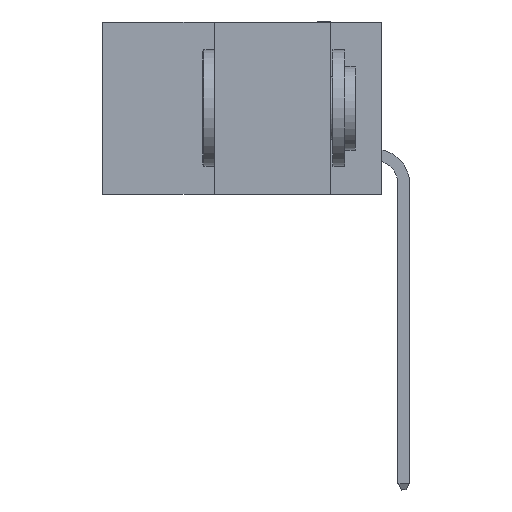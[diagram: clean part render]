
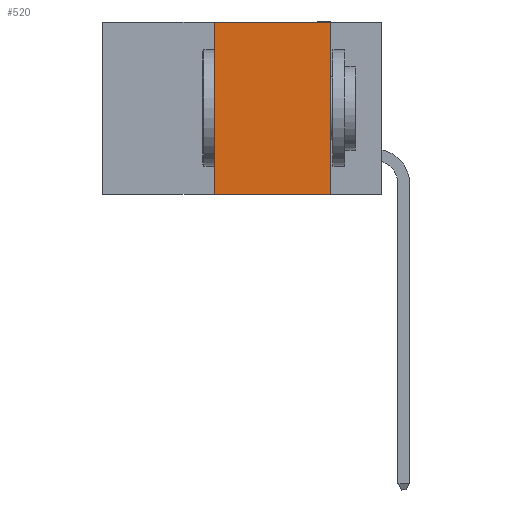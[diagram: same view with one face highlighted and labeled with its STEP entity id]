
A CAD part, left-side view. The second image highlights one B-rep face of the part: STEP entity #520.
In plain terms, the highlighted planar face has unit normal (-1, 0, 0).
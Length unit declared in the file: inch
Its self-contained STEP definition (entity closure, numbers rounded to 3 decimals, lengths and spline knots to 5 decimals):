
#33 = VECTOR ( 'NONE', #3476, 39.37008 ) ;
#520 = ADVANCED_FACE ( 'NONE', ( #874 ), #20718, .F. ) ;
#874 = FACE_OUTER_BOUND ( 'NONE', #17582, .T. ) ;
#1831 = EDGE_CURVE ( 'NONE', #6758, #14218, #6035, .T. ) ;
#2792 = CARTESIAN_POINT ( 'NONE',  ( 0., 0.6, 0. ) ) ;
#3294 = DIRECTION ( 'NONE',  ( 0., 0., -1. ) ) ;
#3476 = DIRECTION ( 'NONE',  ( 0., 0., 1. ) ) ;
#3549 = CARTESIAN_POINT ( 'NONE',  ( 0., 0.36, 0. ) ) ;
#5168 = VECTOR ( 'NONE', #14401, 39.37008 ) ;
#5450 = CARTESIAN_POINT ( 'NONE',  ( 0., 0.6, -0.37 ) ) ;
#6035 = LINE ( 'NONE', #3549, #33 ) ;
#6758 = VERTEX_POINT ( 'NONE', #16211 ) ;
#6889 = DIRECTION ( 'NONE',  ( 0., -1., 0. ) ) ;
#7067 = LINE ( 'NONE', #20879, #9161 ) ;
#7199 = ORIENTED_EDGE ( 'NONE', *, *, #16584, .F. ) ;
#7770 = CARTESIAN_POINT ( 'NONE',  ( 0., 0.6, 0. ) ) ;
#8630 = CARTESIAN_POINT ( 'NONE',  ( 0., 0.11, 0. ) ) ;
#9161 = VECTOR ( 'NONE', #3294, 39.37008 ) ;
#9444 = CARTESIAN_POINT ( 'NONE',  ( 0., 0.36, 0. ) ) ;
#10994 = DIRECTION ( 'NONE',  ( 0., 0., -1. ) ) ;
#13153 = EDGE_CURVE ( 'NONE', #16116, #20457, #7067, .T. ) ;
#13421 = LINE ( 'NONE', #5450, #20558 ) ;
#14218 = VERTEX_POINT ( 'NONE', #9444 ) ;
#14401 = DIRECTION ( 'NONE',  ( 0., -1., 0. ) ) ;
#14456 = AXIS2_PLACEMENT_3D ( 'NONE', #7770, #15873, #10994 ) ;
#15873 = DIRECTION ( 'NONE',  ( 1., 0., 0. ) ) ;
#16116 = VERTEX_POINT ( 'NONE', #8630 ) ;
#16211 = CARTESIAN_POINT ( 'NONE',  ( 0., 0.36, -0.37 ) ) ;
#16520 = ORIENTED_EDGE ( 'NONE', *, *, #1831, .F. ) ;
#16584 = EDGE_CURVE ( 'NONE', #14218, #16116, #19816, .T. ) ;
#16678 = EDGE_CURVE ( 'NONE', #6758, #20457, #13421, .T. ) ;
#17582 = EDGE_LOOP ( 'NONE', ( #18427, #7199, #16520, #18396 ) ) ;
#17916 = CARTESIAN_POINT ( 'NONE',  ( 0., 0.11, -0.37 ) ) ;
#18396 = ORIENTED_EDGE ( 'NONE', *, *, #16678, .T. ) ;
#18427 = ORIENTED_EDGE ( 'NONE', *, *, #13153, .F. ) ;
#19816 = LINE ( 'NONE', #2792, #5168 ) ;
#20457 = VERTEX_POINT ( 'NONE', #17916 ) ;
#20558 = VECTOR ( 'NONE', #6889, 39.37008 ) ;
#20718 = PLANE ( 'NONE',  #14456 ) ;
#20879 = CARTESIAN_POINT ( 'NONE',  ( 0., 0.11, 0. ) ) ;
